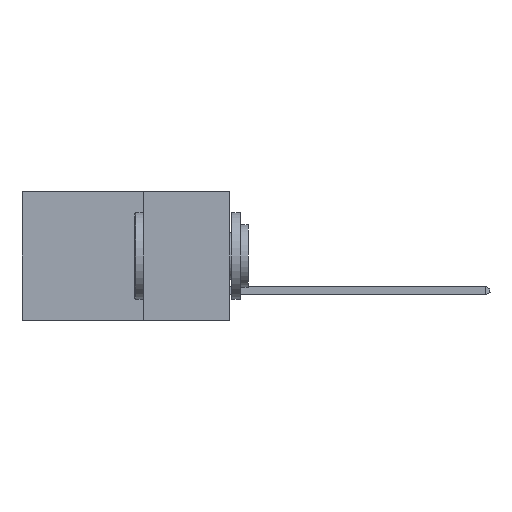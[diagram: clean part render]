
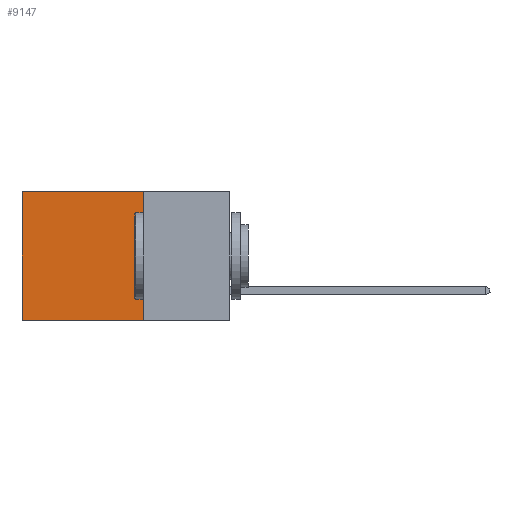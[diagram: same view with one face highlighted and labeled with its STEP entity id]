
A CAD part, left-side view. The second image highlights one B-rep face of the part: STEP entity #9147.
In plain terms, the highlighted planar face has unit normal (-1, 0, 0).
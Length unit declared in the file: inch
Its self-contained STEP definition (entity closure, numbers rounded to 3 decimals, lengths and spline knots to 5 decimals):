
#314 = PLANE ( 'NONE',  #17586 ) ;
#762 = CARTESIAN_POINT ( 'NONE',  ( 0.298, 0.25, 0. ) ) ;
#863 = EDGE_CURVE ( 'NONE', #8801, #15646, #3937, .T. ) ;
#1346 = FACE_OUTER_BOUND ( 'NONE', #12780, .T. ) ;
#1735 = EDGE_CURVE ( 'NONE', #9977, #10532, #5321, .T. ) ;
#2666 = DIRECTION ( 'NONE',  ( 0., 0., -1. ) ) ;
#3694 = EDGE_CURVE ( 'NONE', #9977, #8801, #15401, .T. ) ;
#3937 = LINE ( 'NONE', #4906, #22218 ) ;
#4488 = CARTESIAN_POINT ( 'NONE',  ( 0.298, 0.6, -0.37 ) ) ;
#4906 = CARTESIAN_POINT ( 'NONE',  ( 0.298, 0.25, -0.37 ) ) ;
#5321 = LINE ( 'NONE', #17325, #12079 ) ;
#7152 = LINE ( 'NONE', #9807, #20900 ) ;
#8801 = VERTEX_POINT ( 'NONE', #9444 ) ;
#9147 = ADVANCED_FACE ( 'NONE', ( #1346 ), #314, .F. ) ;
#9444 = CARTESIAN_POINT ( 'NONE',  ( 0.298, 0.25, -0.37 ) ) ;
#9807 = CARTESIAN_POINT ( 'NONE',  ( 0.298, 0.6, 0. ) ) ;
#9977 = VERTEX_POINT ( 'NONE', #12582 ) ;
#10336 = DIRECTION ( 'NONE',  ( 0., 1., 0. ) ) ;
#10532 = VERTEX_POINT ( 'NONE', #15650 ) ;
#11104 = CARTESIAN_POINT ( 'NONE',  ( 0.298, 0.25, 0. ) ) ;
#11619 = DIRECTION ( 'NONE',  ( 0., 0., -1. ) ) ;
#12079 = VECTOR ( 'NONE', #15385, 39.37008 ) ;
#12582 = CARTESIAN_POINT ( 'NONE',  ( 0.298, 0.25, 0. ) ) ;
#12780 = EDGE_LOOP ( 'NONE', ( #20202, #20291, #18993, #19586 ) ) ;
#12936 = DIRECTION ( 'NONE',  ( 1., 0., 0. ) ) ;
#15385 = DIRECTION ( 'NONE',  ( 0., 1., 0. ) ) ;
#15401 = LINE ( 'NONE', #762, #21811 ) ;
#15646 = VERTEX_POINT ( 'NONE', #4488 ) ;
#15650 = CARTESIAN_POINT ( 'NONE',  ( 0.298, 0.6, 0. ) ) ;
#17325 = CARTESIAN_POINT ( 'NONE',  ( 0.298, 0.25, 0. ) ) ;
#17586 = AXIS2_PLACEMENT_3D ( 'NONE', #11104, #12936, #23273 ) ;
#18993 = ORIENTED_EDGE ( 'NONE', *, *, #3694, .F. ) ;
#19586 = ORIENTED_EDGE ( 'NONE', *, *, #1735, .T. ) ;
#20202 = ORIENTED_EDGE ( 'NONE', *, *, #20614, .T. ) ;
#20291 = ORIENTED_EDGE ( 'NONE', *, *, #863, .F. ) ;
#20614 = EDGE_CURVE ( 'NONE', #10532, #15646, #7152, .T. ) ;
#20900 = VECTOR ( 'NONE', #11619, 39.37008 ) ;
#21811 = VECTOR ( 'NONE', #2666, 39.37008 ) ;
#22218 = VECTOR ( 'NONE', #10336, 39.37008 ) ;
#23273 = DIRECTION ( 'NONE',  ( 0., 0., -1. ) ) ;
